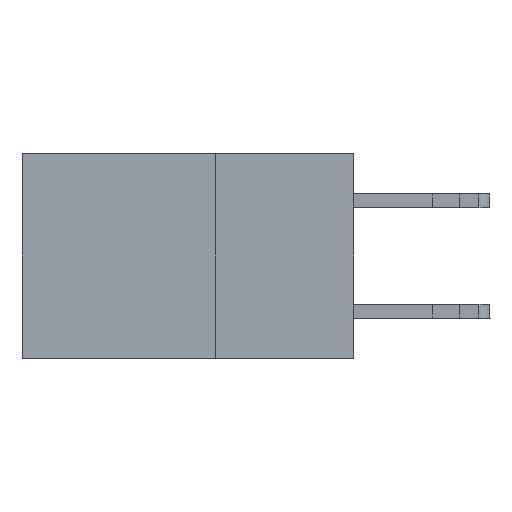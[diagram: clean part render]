
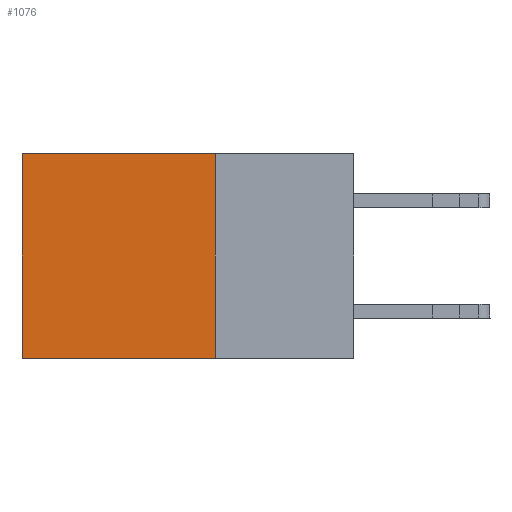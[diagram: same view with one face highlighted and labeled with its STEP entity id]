
A CAD part, left-side view. The second image highlights one B-rep face of the part: STEP entity #1076.
In plain terms, the highlighted planar face has unit normal (-1, 0, 0).
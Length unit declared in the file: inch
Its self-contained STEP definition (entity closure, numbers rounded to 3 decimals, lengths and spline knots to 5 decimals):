
#846 = DIRECTION ( 'NONE',  ( 0., 1., 0. ) ) ;
#1076 = ADVANCED_FACE ( 'NONE', ( #28707 ), #2556, .F. ) ;
#1963 = VECTOR ( 'NONE', #29885, 39.37008 ) ;
#2206 = EDGE_CURVE ( 'NONE', #6778, #29339, #3198, .T. ) ;
#2338 = CARTESIAN_POINT ( 'NONE',  ( 0.2875, 0.25, 0. ) ) ;
#2556 = PLANE ( 'NONE',  #24423 ) ;
#3198 = LINE ( 'NONE', #21895, #25042 ) ;
#3832 = LINE ( 'NONE', #13585, #10463 ) ;
#3915 = DIRECTION ( 'NONE',  ( 0., 1., 0. ) ) ;
#4100 = ORIENTED_EDGE ( 'NONE', *, *, #30221, .F. ) ;
#4173 = VERTEX_POINT ( 'NONE', #24594 ) ;
#4843 = VERTEX_POINT ( 'NONE', #5644 ) ;
#4977 = DIRECTION ( 'NONE',  ( 0., 0., -1. ) ) ;
#5644 = CARTESIAN_POINT ( 'NONE',  ( 0.2875, 0.25, 0. ) ) ;
#5763 = CARTESIAN_POINT ( 'NONE',  ( 0.2875, 0.6, -0.37 ) ) ;
#6778 = VERTEX_POINT ( 'NONE', #23333 ) ;
#9414 = DIRECTION ( 'NONE',  ( 0., 0., -1. ) ) ;
#10463 = VECTOR ( 'NONE', #846, 39.37008 ) ;
#12422 = CARTESIAN_POINT ( 'NONE',  ( 0.2875, 0.25, 0. ) ) ;
#12997 = EDGE_CURVE ( 'NONE', #4843, #6778, #30590, .T. ) ;
#13585 = CARTESIAN_POINT ( 'NONE',  ( 0.2875, 0.25, -0.37 ) ) ;
#14035 = LINE ( 'NONE', #12422, #1963 ) ;
#19076 = CARTESIAN_POINT ( 'NONE',  ( 0.2875, 0.25, 0. ) ) ;
#19887 = DIRECTION ( 'NONE',  ( 1., 0., 0. ) ) ;
#21053 = ORIENTED_EDGE ( 'NONE', *, *, #12997, .T. ) ;
#21895 = CARTESIAN_POINT ( 'NONE',  ( 0.2875, 0.6, 0. ) ) ;
#23333 = CARTESIAN_POINT ( 'NONE',  ( 0.2875, 0.6, 0. ) ) ;
#23421 = EDGE_CURVE ( 'NONE', #4173, #29339, #3832, .T. ) ;
#23539 = ORIENTED_EDGE ( 'NONE', *, *, #2206, .T. ) ;
#24423 = AXIS2_PLACEMENT_3D ( 'NONE', #2338, #19887, #4977 ) ;
#24594 = CARTESIAN_POINT ( 'NONE',  ( 0.2875, 0.25, -0.37 ) ) ;
#25042 = VECTOR ( 'NONE', #9414, 39.37008 ) ;
#25122 = VECTOR ( 'NONE', #3915, 39.37008 ) ;
#26623 = EDGE_LOOP ( 'NONE', ( #23539, #31752, #4100, #21053 ) ) ;
#28707 = FACE_OUTER_BOUND ( 'NONE', #26623, .T. ) ;
#29339 = VERTEX_POINT ( 'NONE', #5763 ) ;
#29885 = DIRECTION ( 'NONE',  ( 0., 0., -1. ) ) ;
#30221 = EDGE_CURVE ( 'NONE', #4843, #4173, #14035, .T. ) ;
#30590 = LINE ( 'NONE', #19076, #25122 ) ;
#31752 = ORIENTED_EDGE ( 'NONE', *, *, #23421, .F. ) ;
